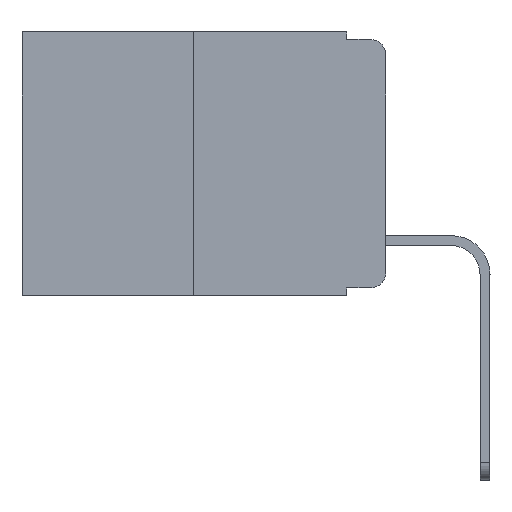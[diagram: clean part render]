
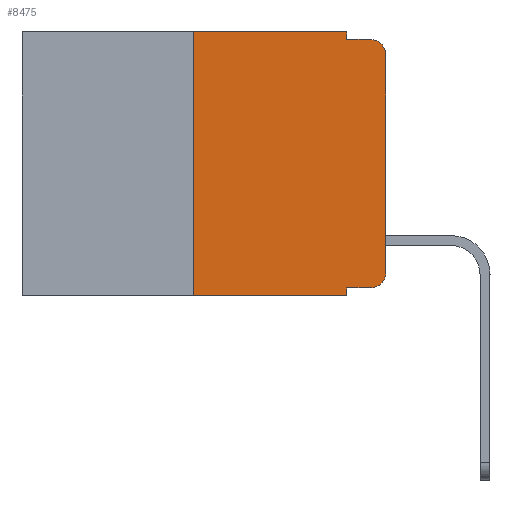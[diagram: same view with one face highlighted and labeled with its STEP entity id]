
A CAD part, left-side view. The second image highlights one B-rep face of the part: STEP entity #8475.
In plain terms, the highlighted planar face has unit normal (-1, 0, 0).
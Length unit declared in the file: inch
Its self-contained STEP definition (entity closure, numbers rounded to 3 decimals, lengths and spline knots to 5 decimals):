
#86 = VECTOR ( 'NONE', #3449, 39.37008 ) ;
#293 = ORIENTED_EDGE ( 'NONE', *, *, #13571, .T. ) ;
#311 = LINE ( 'NONE', #8950, #86 ) ;
#318 = EDGE_CURVE ( 'NONE', #13100, #15231, #311, .T. ) ;
#619 = VECTOR ( 'NONE', #6243, 39.37008 ) ;
#689 = LINE ( 'NONE', #11490, #7483 ) ;
#694 = CARTESIAN_POINT ( 'NONE',  ( 0., 0.473, -0.343 ) ) ;
#746 = LINE ( 'NONE', #4286, #9232 ) ;
#1925 = VECTOR ( 'NONE', #8247, 39.37008 ) ;
#2030 = ORIENTED_EDGE ( 'NONE', *, *, #10245, .T. ) ;
#2122 = DIRECTION ( 'NONE',  ( 0., -1., 0. ) ) ;
#2247 = VERTEX_POINT ( 'NONE', #2921 ) ;
#2333 = ORIENTED_EDGE ( 'NONE', *, *, #4663, .T. ) ;
#2361 = EDGE_CURVE ( 'NONE', #13100, #5805, #12691, .T. ) ;
#2559 = CARTESIAN_POINT ( 'NONE',  ( 0., 0.02, -0.313 ) ) ;
#2895 = DIRECTION ( 'NONE',  ( 0., 0., 1. ) ) ;
#2921 = CARTESIAN_POINT ( 'NONE',  ( 0., 0.25, -0.343 ) ) ;
#3218 = CARTESIAN_POINT ( 'NONE',  ( 0., 0., -0.03 ) ) ;
#3388 = LINE ( 'NONE', #7720, #619 ) ;
#3449 = DIRECTION ( 'NONE',  ( 0., 0., -1. ) ) ;
#3522 = PLANE ( 'NONE',  #15400 ) ;
#3590 = LINE ( 'NONE', #10685, #9512 ) ;
#4286 = CARTESIAN_POINT ( 'NONE',  ( 0., 0.25, 0. ) ) ;
#4663 = EDGE_CURVE ( 'NONE', #10546, #9314, #8451, .T. ) ;
#4775 = DIRECTION ( 'NONE',  ( 1., 0., 0. ) ) ;
#4836 = AXIS2_PLACEMENT_3D ( 'NONE', #13814, #12308, #5789 ) ;
#5536 = ORIENTED_EDGE ( 'NONE', *, *, #318, .F. ) ;
#5718 = ORIENTED_EDGE ( 'NONE', *, *, #11851, .F. ) ;
#5729 = CARTESIAN_POINT ( 'NONE',  ( 0., 0.25, 0. ) ) ;
#5789 = DIRECTION ( 'NONE',  ( 0., 0., -1. ) ) ;
#5805 = VERTEX_POINT ( 'NONE', #6505 ) ;
#5867 = CARTESIAN_POINT ( 'NONE',  ( 0., 0.051, -0.01 ) ) ;
#6243 = DIRECTION ( 'NONE',  ( 0., 0., -1. ) ) ;
#6460 = ORIENTED_EDGE ( 'NONE', *, *, #10348, .F. ) ;
#6505 = CARTESIAN_POINT ( 'NONE',  ( 0., 0.02, -0.333 ) ) ;
#7465 = CARTESIAN_POINT ( 'NONE',  ( 0., 0.051, 0. ) ) ;
#7483 = VECTOR ( 'NONE', #11437, 39.37008 ) ;
#7559 = CARTESIAN_POINT ( 'NONE',  ( 0., 0., -0.313 ) ) ;
#7560 = VECTOR ( 'NONE', #2895, 39.37008 ) ;
#7574 = CARTESIAN_POINT ( 'NONE',  ( 0., 0.051, -0.333 ) ) ;
#7720 = CARTESIAN_POINT ( 'NONE',  ( 0., 0.051, 0. ) ) ;
#7833 = EDGE_CURVE ( 'NONE', #2247, #15231, #15619, .T. ) ;
#7844 = AXIS2_PLACEMENT_3D ( 'NONE', #2559, #13221, #15895 ) ;
#8247 = DIRECTION ( 'NONE',  ( 0., -1., 0. ) ) ;
#8451 = CIRCLE ( 'NONE', #4836, 0.02 ) ;
#8475 = ADVANCED_FACE ( 'NONE', ( #10112 ), #3522, .F. ) ;
#8541 = ORIENTED_EDGE ( 'NONE', *, *, #11387, .F. ) ;
#8950 = CARTESIAN_POINT ( 'NONE',  ( 0., 0.051, 0. ) ) ;
#9232 = VECTOR ( 'NONE', #13623, 39.37008 ) ;
#9314 = VERTEX_POINT ( 'NONE', #13322 ) ;
#9512 = VECTOR ( 'NONE', #14771, 39.37008 ) ;
#9587 = VERTEX_POINT ( 'NONE', #5867 ) ;
#9621 = CARTESIAN_POINT ( 'NONE',  ( 0., 0., 0. ) ) ;
#9647 = CIRCLE ( 'NONE', #7844, 0.02 ) ;
#10112 = FACE_OUTER_BOUND ( 'NONE', #11928, .T. ) ;
#10245 = EDGE_CURVE ( 'NONE', #5805, #15580, #9647, .T. ) ;
#10348 = EDGE_CURVE ( 'NONE', #2247, #14132, #746, .T. ) ;
#10546 = VERTEX_POINT ( 'NONE', #3218 ) ;
#10685 = CARTESIAN_POINT ( 'NONE',  ( 0., 0.051, -0.01 ) ) ;
#11050 = ORIENTED_EDGE ( 'NONE', *, *, #2361, .T. ) ;
#11387 = EDGE_CURVE ( 'NONE', #9587, #9314, #3590, .T. ) ;
#11437 = DIRECTION ( 'NONE',  ( 0., -1., 0. ) ) ;
#11490 = CARTESIAN_POINT ( 'NONE',  ( 0., 0.473, 0. ) ) ;
#11605 = CARTESIAN_POINT ( 'NONE',  ( 0., 0.473, 0. ) ) ;
#11851 = EDGE_CURVE ( 'NONE', #13186, #9587, #3388, .T. ) ;
#11928 = EDGE_LOOP ( 'NONE', ( #293, #2333, #8541, #5718, #16078, #6460, #14682, #5536, #11050, #2030 ) ) ;
#12308 = DIRECTION ( 'NONE',  ( -1., 0., 0. ) ) ;
#12691 = LINE ( 'NONE', #16301, #1925 ) ;
#13100 = VERTEX_POINT ( 'NONE', #7574 ) ;
#13186 = VERTEX_POINT ( 'NONE', #7465 ) ;
#13221 = DIRECTION ( 'NONE',  ( -1., 0., 0. ) ) ;
#13322 = CARTESIAN_POINT ( 'NONE',  ( 0., 0.02, -0.01 ) ) ;
#13571 = EDGE_CURVE ( 'NONE', #15580, #10546, #14688, .T. ) ;
#13623 = DIRECTION ( 'NONE',  ( 0., 0., 1. ) ) ;
#13814 = CARTESIAN_POINT ( 'NONE',  ( 0., 0.02, -0.03 ) ) ;
#14132 = VERTEX_POINT ( 'NONE', #5729 ) ;
#14682 = ORIENTED_EDGE ( 'NONE', *, *, #7833, .T. ) ;
#14688 = LINE ( 'NONE', #9621, #7560 ) ;
#14771 = DIRECTION ( 'NONE',  ( 0., -1., 0. ) ) ;
#15231 = VERTEX_POINT ( 'NONE', #17322 ) ;
#15400 = AXIS2_PLACEMENT_3D ( 'NONE', #11605, #4775, #16829 ) ;
#15580 = VERTEX_POINT ( 'NONE', #7559 ) ;
#15595 = EDGE_CURVE ( 'NONE', #14132, #13186, #689, .T. ) ;
#15619 = LINE ( 'NONE', #694, #16656 ) ;
#15895 = DIRECTION ( 'NONE',  ( 0., 0., -1. ) ) ;
#16078 = ORIENTED_EDGE ( 'NONE', *, *, #15595, .F. ) ;
#16301 = CARTESIAN_POINT ( 'NONE',  ( 0., 0.051, -0.333 ) ) ;
#16656 = VECTOR ( 'NONE', #2122, 39.37008 ) ;
#16829 = DIRECTION ( 'NONE',  ( 0., 0., -1. ) ) ;
#17322 = CARTESIAN_POINT ( 'NONE',  ( 0., 0.051, -0.343 ) ) ;
